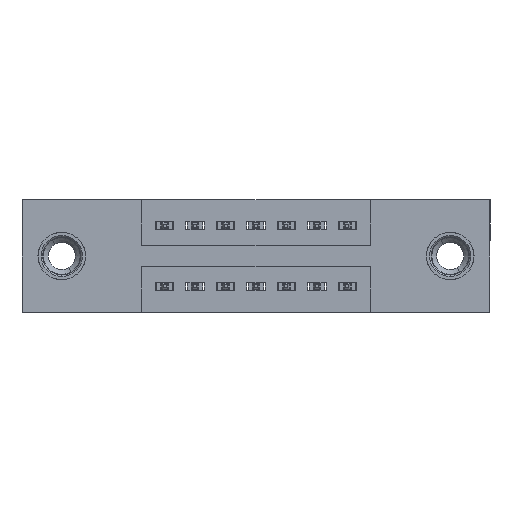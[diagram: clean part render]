
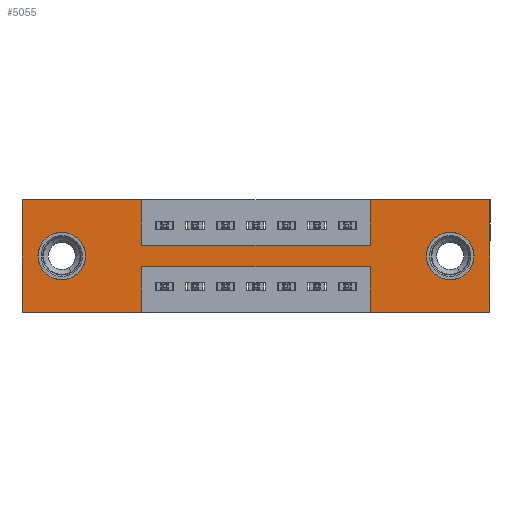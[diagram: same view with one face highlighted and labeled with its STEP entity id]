
A CAD part, front view. The second image highlights one B-rep face of the part: STEP entity #5055.
In plain terms, the highlighted planar face has unit normal (0, -1, 0).
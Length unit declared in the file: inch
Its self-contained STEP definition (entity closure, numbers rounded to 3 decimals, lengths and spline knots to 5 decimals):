
#4 = VECTOR ( 'NONE', #8132, 39.37008 ) ;
#77 = CARTESIAN_POINT ( 'NONE',  ( 1.405, 0., -0.263 ) ) ;
#142 = CARTESIAN_POINT ( 'NONE',  ( 0.3925, 0., 0. ) ) ;
#276 = EDGE_CURVE ( 'NONE', #1372, #1896, #4898, .T. ) ;
#356 = CARTESIAN_POINT ( 'NONE',  ( 1.535, 0., 0. ) ) ;
#387 = AXIS2_PLACEMENT_3D ( 'NONE', #7963, #922, #9108 ) ;
#602 = AXIS2_PLACEMENT_3D ( 'NONE', #961, #9152, #2244 ) ;
#630 = VERTEX_POINT ( 'NONE', #5798 ) ;
#719 = EDGE_CURVE ( 'NONE', #1868, #1372, #2503, .T. ) ;
#875 = VERTEX_POINT ( 'NONE', #10053 ) ;
#922 = DIRECTION ( 'NONE',  ( 0., 1., 0. ) ) ;
#961 = CARTESIAN_POINT ( 'NONE',  ( 0.13, 0., -0.185 ) ) ;
#1019 = VERTEX_POINT ( 'NONE', #10396 ) ;
#1175 = DIRECTION ( 'NONE',  ( -1., 0., 0. ) ) ;
#1236 = CARTESIAN_POINT ( 'NONE',  ( 0.13, 0., -0.263 ) ) ;
#1270 = CARTESIAN_POINT ( 'NONE',  ( 0.3925, 0., -0.37 ) ) ;
#1325 = DIRECTION ( 'NONE',  ( 0., 0., -1. ) ) ;
#1372 = VERTEX_POINT ( 'NONE', #11481 ) ;
#1560 = AXIS2_PLACEMENT_3D ( 'NONE', #13333, #6548, #14461 ) ;
#1614 = CARTESIAN_POINT ( 'NONE',  ( 0., 0., -0.37 ) ) ;
#1731 = CIRCLE ( 'NONE', #9756, 0.078 ) ;
#1868 = VERTEX_POINT ( 'NONE', #12457 ) ;
#1896 = VERTEX_POINT ( 'NONE', #9920 ) ;
#2206 = EDGE_CURVE ( 'NONE', #1896, #5001, #4508, .T. ) ;
#2244 = DIRECTION ( 'NONE',  ( 0., 0., 1. ) ) ;
#2277 = CARTESIAN_POINT ( 'NONE',  ( 0., 0., 0. ) ) ;
#2317 = PLANE ( 'NONE',  #9505 ) ;
#2363 = DIRECTION ( 'NONE',  ( 0., -1., 0. ) ) ;
#2503 = LINE ( 'NONE', #7292, #14310 ) ;
#2533 = DIRECTION ( 'NONE',  ( 0., 0., 1. ) ) ;
#2617 = CARTESIAN_POINT ( 'NONE',  ( 1.1425, 0., 0. ) ) ;
#2657 = DIRECTION ( 'NONE',  ( 0., 0., -1. ) ) ;
#3130 = EDGE_CURVE ( 'NONE', #8834, #12878, #9306, .T. ) ;
#3158 = FACE_OUTER_BOUND ( 'NONE', #7569, .T. ) ;
#3236 = LINE ( 'NONE', #12504, #11973 ) ;
#3261 = LINE ( 'NONE', #8161, #9711 ) ;
#3327 = LINE ( 'NONE', #10383, #4 ) ;
#3387 = DIRECTION ( 'NONE',  ( 0., 0., 1. ) ) ;
#3466 = CARTESIAN_POINT ( 'NONE',  ( 1.1425, 0., 0. ) ) ;
#3585 = VERTEX_POINT ( 'NONE', #2617 ) ;
#3645 = ORIENTED_EDGE ( 'NONE', *, *, #6845, .T. ) ;
#3696 = ORIENTED_EDGE ( 'NONE', *, *, #12681, .F. ) ;
#3736 = CARTESIAN_POINT ( 'NONE',  ( 0.13, 0., -0.107 ) ) ;
#3755 = ORIENTED_EDGE ( 'NONE', *, *, #14096, .F. ) ;
#3906 = CARTESIAN_POINT ( 'NONE',  ( 0.3925, 0., -0.22 ) ) ;
#4052 = EDGE_CURVE ( 'NONE', #875, #7071, #7331, .T. ) ;
#4215 = ORIENTED_EDGE ( 'NONE', *, *, #2206, .F. ) ;
#4251 = EDGE_LOOP ( 'NONE', ( #4776, #10473 ) ) ;
#4275 = VECTOR ( 'NONE', #13017, 39.37008 ) ;
#4411 = ORIENTED_EDGE ( 'NONE', *, *, #719, .F. ) ;
#4485 = EDGE_CURVE ( 'NONE', #3585, #7291, #10713, .T. ) ;
#4495 = ORIENTED_EDGE ( 'NONE', *, *, #11599, .F. ) ;
#4506 = CARTESIAN_POINT ( 'NONE',  ( 0., 0., 0. ) ) ;
#4508 = LINE ( 'NONE', #12962, #10610 ) ;
#4602 = VERTEX_POINT ( 'NONE', #3736 ) ;
#4620 = VECTOR ( 'NONE', #10389, 39.37008 ) ;
#4776 = ORIENTED_EDGE ( 'NONE', *, *, #9732, .T. ) ;
#4898 = LINE ( 'NONE', #142, #13267 ) ;
#4902 = CARTESIAN_POINT ( 'NONE',  ( 1.405, 0., -0.185 ) ) ;
#4965 = VECTOR ( 'NONE', #2533, 39.37008 ) ;
#5001 = VERTEX_POINT ( 'NONE', #8005 ) ;
#5018 = ORIENTED_EDGE ( 'NONE', *, *, #4052, .F. ) ;
#5055 = ADVANCED_FACE ( 'NONE', ( #12255, #9250, #3158 ), #2317, .T. ) ;
#5775 = ORIENTED_EDGE ( 'NONE', *, *, #6293, .F. ) ;
#5798 = CARTESIAN_POINT ( 'NONE',  ( 1.1425, 0., -0.37 ) ) ;
#5912 = VECTOR ( 'NONE', #1175, 39.37008 ) ;
#6057 = DIRECTION ( 'NONE',  ( 0., 0., -1. ) ) ;
#6080 = VECTOR ( 'NONE', #11479, 39.37008 ) ;
#6265 = ORIENTED_EDGE ( 'NONE', *, *, #10445, .T. ) ;
#6293 = EDGE_CURVE ( 'NONE', #7291, #7180, #3327, .T. ) ;
#6374 = EDGE_LOOP ( 'NONE', ( #6265, #3645 ) ) ;
#6504 = VERTEX_POINT ( 'NONE', #1236 ) ;
#6548 = DIRECTION ( 'NONE',  ( 0., 1., 0. ) ) ;
#6592 = CARTESIAN_POINT ( 'NONE',  ( 0., 0., -0.37 ) ) ;
#6845 = EDGE_CURVE ( 'NONE', #6504, #4602, #14356, .T. ) ;
#7071 = VERTEX_POINT ( 'NONE', #10370 ) ;
#7176 = CARTESIAN_POINT ( 'NONE',  ( 1.535, 0., -0.37 ) ) ;
#7180 = VERTEX_POINT ( 'NONE', #7176 ) ;
#7291 = VERTEX_POINT ( 'NONE', #356 ) ;
#7292 = CARTESIAN_POINT ( 'NONE',  ( 0., 0., 0. ) ) ;
#7331 = LINE ( 'NONE', #3906, #4275 ) ;
#7561 = EDGE_CURVE ( 'NONE', #12878, #1868, #8858, .T. ) ;
#7562 = DIRECTION ( 'NONE',  ( 1., 0., 0. ) ) ;
#7569 = EDGE_LOOP ( 'NONE', ( #13325, #5018, #3696, #3755, #5775, #9978, #4495, #4215, #13813, #4411, #15041, #7845 ) ) ;
#7845 = ORIENTED_EDGE ( 'NONE', *, *, #3130, .F. ) ;
#7963 = CARTESIAN_POINT ( 'NONE',  ( 1.405, 0., -0.185 ) ) ;
#7994 = LINE ( 'NONE', #15060, #4965 ) ;
#8005 = CARTESIAN_POINT ( 'NONE',  ( 1.1425, 0., -0.15 ) ) ;
#8132 = DIRECTION ( 'NONE',  ( 0., 0., -1. ) ) ;
#8161 = CARTESIAN_POINT ( 'NONE',  ( 0.3925, 0., -0.37 ) ) ;
#8834 = VERTEX_POINT ( 'NONE', #1270 ) ;
#8858 = LINE ( 'NONE', #4506, #11486 ) ;
#9100 = LINE ( 'NONE', #3466, #6080 ) ;
#9108 = DIRECTION ( 'NONE',  ( 0., 0., -1. ) ) ;
#9152 = DIRECTION ( 'NONE',  ( 0., 1., 0. ) ) ;
#9250 = FACE_BOUND ( 'NONE', #6374, .T. ) ;
#9262 = CARTESIAN_POINT ( 'NONE',  ( 0., 0., -0.37 ) ) ;
#9306 = LINE ( 'NONE', #6592, #5912 ) ;
#9505 = AXIS2_PLACEMENT_3D ( 'NONE', #9262, #2363, #10425 ) ;
#9711 = VECTOR ( 'NONE', #1325, 39.37008 ) ;
#9732 = EDGE_CURVE ( 'NONE', #1019, #9985, #14130, .T. ) ;
#9756 = AXIS2_PLACEMENT_3D ( 'NONE', #4902, #12862, #6057 ) ;
#9920 = CARTESIAN_POINT ( 'NONE',  ( 0.3925, 0., -0.15 ) ) ;
#9978 = ORIENTED_EDGE ( 'NONE', *, *, #4485, .F. ) ;
#9985 = VERTEX_POINT ( 'NONE', #77 ) ;
#10053 = CARTESIAN_POINT ( 'NONE',  ( 1.1425, 0., -0.22 ) ) ;
#10370 = CARTESIAN_POINT ( 'NONE',  ( 0.3925, 0., -0.22 ) ) ;
#10383 = CARTESIAN_POINT ( 'NONE',  ( 1.535, 0., 0. ) ) ;
#10389 = DIRECTION ( 'NONE',  ( 1., 0., 0. ) ) ;
#10396 = CARTESIAN_POINT ( 'NONE',  ( 1.405, 0., -0.107 ) ) ;
#10425 = DIRECTION ( 'NONE',  ( 0., 0., -1. ) ) ;
#10445 = EDGE_CURVE ( 'NONE', #4602, #6504, #11600, .T. ) ;
#10473 = ORIENTED_EDGE ( 'NONE', *, *, #13747, .T. ) ;
#10610 = VECTOR ( 'NONE', #11733, 39.37008 ) ;
#10713 = LINE ( 'NONE', #2277, #4620 ) ;
#11479 = DIRECTION ( 'NONE',  ( 0., 0., 1. ) ) ;
#11481 = CARTESIAN_POINT ( 'NONE',  ( 0.3925, 0., 0. ) ) ;
#11486 = VECTOR ( 'NONE', #3387, 39.37008 ) ;
#11599 = EDGE_CURVE ( 'NONE', #5001, #3585, #9100, .T. ) ;
#11600 = CIRCLE ( 'NONE', #602, 0.078 ) ;
#11733 = DIRECTION ( 'NONE',  ( 1., 0., 0. ) ) ;
#11973 = VECTOR ( 'NONE', #14721, 39.37008 ) ;
#12255 = FACE_BOUND ( 'NONE', #4251, .T. ) ;
#12457 = CARTESIAN_POINT ( 'NONE',  ( 0., 0., 0. ) ) ;
#12504 = CARTESIAN_POINT ( 'NONE',  ( 0., 0., -0.37 ) ) ;
#12681 = EDGE_CURVE ( 'NONE', #630, #875, #7994, .T. ) ;
#12862 = DIRECTION ( 'NONE',  ( 0., 1., 0. ) ) ;
#12878 = VERTEX_POINT ( 'NONE', #1614 ) ;
#12962 = CARTESIAN_POINT ( 'NONE',  ( 0.3925, 0., -0.15 ) ) ;
#13017 = DIRECTION ( 'NONE',  ( -1., 0., 0. ) ) ;
#13186 = EDGE_CURVE ( 'NONE', #7071, #8834, #3261, .T. ) ;
#13267 = VECTOR ( 'NONE', #2657, 39.37008 ) ;
#13325 = ORIENTED_EDGE ( 'NONE', *, *, #13186, .F. ) ;
#13333 = CARTESIAN_POINT ( 'NONE',  ( 0.13, 0., -0.185 ) ) ;
#13747 = EDGE_CURVE ( 'NONE', #9985, #1019, #1731, .T. ) ;
#13813 = ORIENTED_EDGE ( 'NONE', *, *, #276, .F. ) ;
#14096 = EDGE_CURVE ( 'NONE', #7180, #630, #3236, .T. ) ;
#14130 = CIRCLE ( 'NONE', #387, 0.078 ) ;
#14310 = VECTOR ( 'NONE', #7562, 39.37008 ) ;
#14356 = CIRCLE ( 'NONE', #1560, 0.078 ) ;
#14461 = DIRECTION ( 'NONE',  ( 0., 0., 1. ) ) ;
#14721 = DIRECTION ( 'NONE',  ( -1., 0., 0. ) ) ;
#15041 = ORIENTED_EDGE ( 'NONE', *, *, #7561, .F. ) ;
#15060 = CARTESIAN_POINT ( 'NONE',  ( 1.1425, 0., -0.37 ) ) ;
